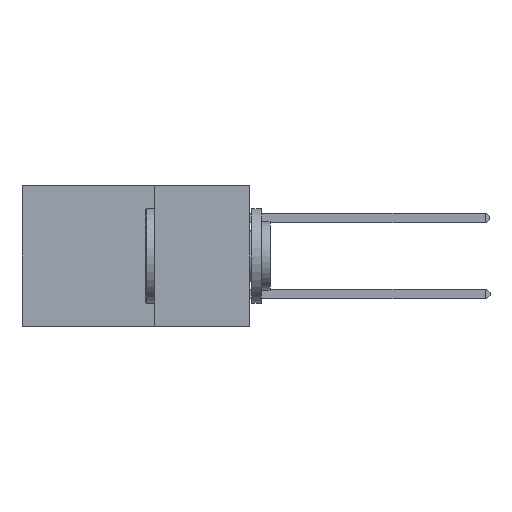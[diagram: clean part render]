
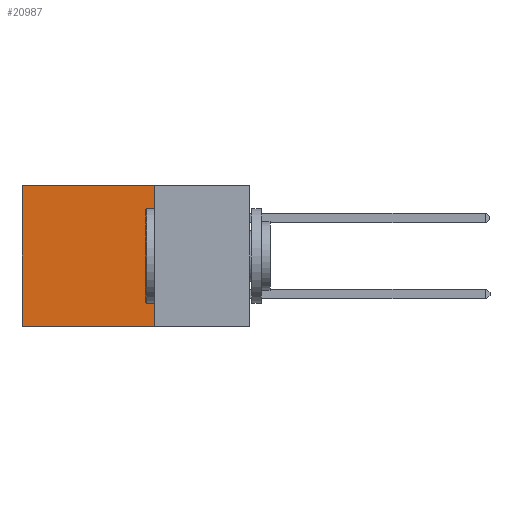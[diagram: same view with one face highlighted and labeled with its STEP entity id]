
A CAD part, left-side view. The second image highlights one B-rep face of the part: STEP entity #20987.
In plain terms, the highlighted planar face has unit normal (-1, 0, 0).
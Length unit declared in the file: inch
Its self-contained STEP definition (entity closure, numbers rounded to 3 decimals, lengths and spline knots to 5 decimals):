
#565 = CARTESIAN_POINT ( 'NONE',  ( 0.2875, 0.25, 0. ) ) ;
#1863 = ORIENTED_EDGE ( 'NONE', *, *, #14952, .T. ) ;
#2407 = PLANE ( 'NONE',  #21246 ) ;
#2807 = LINE ( 'NONE', #16599, #7050 ) ;
#3610 = LINE ( 'NONE', #16145, #12567 ) ;
#3652 = DIRECTION ( 'NONE',  ( 0., 0., -1. ) ) ;
#3770 = CARTESIAN_POINT ( 'NONE',  ( 0.2875, 0.25, -0.37 ) ) ;
#4085 = CARTESIAN_POINT ( 'NONE',  ( 0.2875, 0.6, 0. ) ) ;
#5579 = EDGE_LOOP ( 'NONE', ( #20254, #9699, #20493, #1863 ) ) ;
#5910 = DIRECTION ( 'NONE',  ( 0., 0., -1. ) ) ;
#6085 = DIRECTION ( 'NONE',  ( 1., 0., 0. ) ) ;
#6250 = LINE ( 'NONE', #4085, #15139 ) ;
#6356 = CARTESIAN_POINT ( 'NONE',  ( 0.2875, 0.25, -0.37 ) ) ;
#7050 = VECTOR ( 'NONE', #13016, 39.37008 ) ;
#7109 = VECTOR ( 'NONE', #16253, 39.37008 ) ;
#8934 = VERTEX_POINT ( 'NONE', #10771 ) ;
#9699 = ORIENTED_EDGE ( 'NONE', *, *, #13063, .F. ) ;
#10771 = CARTESIAN_POINT ( 'NONE',  ( 0.2875, 0.25, 0. ) ) ;
#12567 = VECTOR ( 'NONE', #3652, 39.37008 ) ;
#13016 = DIRECTION ( 'NONE',  ( 0., 1., 0. ) ) ;
#13063 = EDGE_CURVE ( 'NONE', #21592, #22716, #19646, .T. ) ;
#13700 = EDGE_CURVE ( 'NONE', #18198, #22716, #6250, .T. ) ;
#14638 = CARTESIAN_POINT ( 'NONE',  ( 0.2875, 0.6, -0.37 ) ) ;
#14952 = EDGE_CURVE ( 'NONE', #8934, #18198, #2807, .T. ) ;
#15139 = VECTOR ( 'NONE', #5910, 39.37008 ) ;
#15686 = FACE_OUTER_BOUND ( 'NONE', #5579, .T. ) ;
#16112 = EDGE_CURVE ( 'NONE', #8934, #21592, #3610, .T. ) ;
#16145 = CARTESIAN_POINT ( 'NONE',  ( 0.2875, 0.25, 0. ) ) ;
#16253 = DIRECTION ( 'NONE',  ( 0., 1., 0. ) ) ;
#16599 = CARTESIAN_POINT ( 'NONE',  ( 0.2875, 0.25, 0. ) ) ;
#18198 = VERTEX_POINT ( 'NONE', #20856 ) ;
#18548 = DIRECTION ( 'NONE',  ( 0., 0., -1. ) ) ;
#19646 = LINE ( 'NONE', #3770, #7109 ) ;
#20254 = ORIENTED_EDGE ( 'NONE', *, *, #13700, .T. ) ;
#20493 = ORIENTED_EDGE ( 'NONE', *, *, #16112, .F. ) ;
#20856 = CARTESIAN_POINT ( 'NONE',  ( 0.2875, 0.6, 0. ) ) ;
#20987 = ADVANCED_FACE ( 'NONE', ( #15686 ), #2407, .F. ) ;
#21246 = AXIS2_PLACEMENT_3D ( 'NONE', #565, #6085, #18548 ) ;
#21592 = VERTEX_POINT ( 'NONE', #6356 ) ;
#22716 = VERTEX_POINT ( 'NONE', #14638 ) ;
